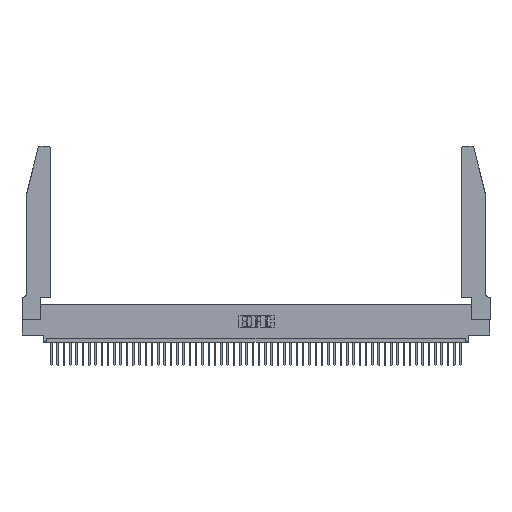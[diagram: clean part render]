
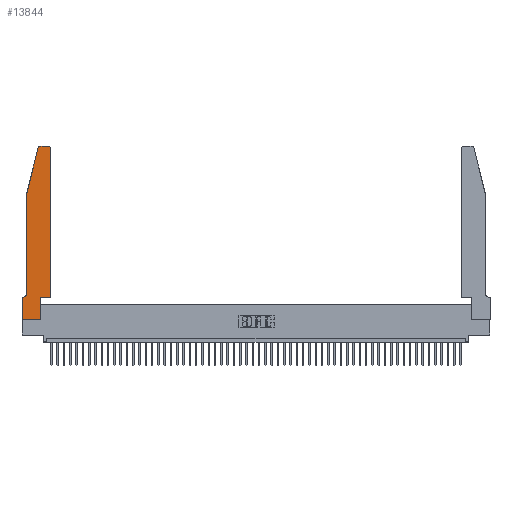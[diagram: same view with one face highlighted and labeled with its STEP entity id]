
A CAD part, top view. The second image highlights one B-rep face of the part: STEP entity #13844.
In plain terms, the highlighted planar face has unit normal (0, 0, 1).
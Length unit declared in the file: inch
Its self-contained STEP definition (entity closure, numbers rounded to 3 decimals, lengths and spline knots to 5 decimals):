
#1140 = VECTOR ( 'NONE', #16106, 39.37008 ) ;
#1264 = VERTEX_POINT ( 'NONE', #22103 ) ;
#1305 = DIRECTION ( 'NONE',  ( 0., 1., 0. ) ) ;
#1679 = CARTESIAN_POINT ( 'NONE',  ( 0.0755, 2., 0.37 ) ) ;
#2089 = DIRECTION ( 'NONE',  ( 0., 0., 1. ) ) ;
#2169 = DIRECTION ( 'NONE',  ( -1., 0., 0. ) ) ;
#2208 = DIRECTION ( 'NONE',  ( 0., 0., 1. ) ) ;
#2503 = VECTOR ( 'NONE', #2169, 39.37008 ) ;
#2646 = ORIENTED_EDGE ( 'NONE', *, *, #10434, .T. ) ;
#3497 = VERTEX_POINT ( 'NONE', #5968 ) ;
#3773 = DIRECTION ( 'NONE',  ( -1., 0., 0. ) ) ;
#3814 = ORIENTED_EDGE ( 'NONE', *, *, #42274, .T. ) ;
#4994 = VECTOR ( 'NONE', #3773, 39.37008 ) ;
#5667 = ORIENTED_EDGE ( 'NONE', *, *, #31963, .T. ) ;
#5926 = VERTEX_POINT ( 'NONE', #17185 ) ;
#5968 = CARTESIAN_POINT ( 'NONE',  ( 0., 0.35, 0.37 ) ) ;
#6052 = VERTEX_POINT ( 'NONE', #27589 ) ;
#6230 = VERTEX_POINT ( 'NONE', #17144 ) ;
#6250 = DIRECTION ( 'NONE',  ( 1., 0., 0. ) ) ;
#6266 = DIRECTION ( 'NONE',  ( 1., 0., 0. ) ) ;
#6328 = ORIENTED_EDGE ( 'NONE', *, *, #15241, .T. ) ;
#6505 = CARTESIAN_POINT ( 'NONE',  ( 0.2865, 0.35, 0.37 ) ) ;
#7185 = ORIENTED_EDGE ( 'NONE', *, *, #11481, .T. ) ;
#7549 = LINE ( 'NONE', #36276, #19295 ) ;
#8269 = ORIENTED_EDGE ( 'NONE', *, *, #35751, .T. ) ;
#8461 = EDGE_CURVE ( 'NONE', #5926, #13390, #28843, .T. ) ;
#9379 = CARTESIAN_POINT ( 'NONE',  ( 0.4505, 0.35, 0.37 ) ) ;
#10176 = VECTOR ( 'NONE', #50410, 39.37008 ) ;
#10383 = FACE_OUTER_BOUND ( 'NONE', #32331, .T. ) ;
#10434 = EDGE_CURVE ( 'NONE', #6052, #14651, #46537, .T. ) ;
#10548 = CARTESIAN_POINT ( 'NONE',  ( 0.4505, 0.35, 0.37 ) ) ;
#11481 = EDGE_CURVE ( 'NONE', #6230, #17994, #36032, .T. ) ;
#12273 = EDGE_CURVE ( 'NONE', #17994, #3497, #48941, .T. ) ;
#13036 = EDGE_CURVE ( 'NONE', #26309, #51332, #46368, .T. ) ;
#13390 = VERTEX_POINT ( 'NONE', #35674 ) ;
#13400 = VECTOR ( 'NONE', #46387, 39.37008 ) ;
#13844 = ADVANCED_FACE ( 'NONE', ( #10383 ), #34217, .T. ) ;
#13885 = ORIENTED_EDGE ( 'NONE', *, *, #8461, .T. ) ;
#14651 = VERTEX_POINT ( 'NONE', #30762 ) ;
#14690 = CARTESIAN_POINT ( 'NONE',  ( 0.0755, 2., 0.37 ) ) ;
#15241 = EDGE_CURVE ( 'NONE', #1264, #6230, #45476, .T. ) ;
#15530 = CARTESIAN_POINT ( 'NONE',  ( 0.2605, 2.75, 0.37 ) ) ;
#16106 = DIRECTION ( 'NONE',  ( 0., 1., 0. ) ) ;
#16199 = DIRECTION ( 'NONE',  ( 1., 0., 0. ) ) ;
#16653 = AXIS2_PLACEMENT_3D ( 'NONE', #29723, #2208, #18300 ) ;
#16791 = AXIS2_PLACEMENT_3D ( 'NONE', #39643, #2089, #6266 ) ;
#17144 = CARTESIAN_POINT ( 'NONE',  ( 0.0755, 0.42, 0.37 ) ) ;
#17185 = CARTESIAN_POINT ( 'NONE',  ( 0.4505, 2.72, 0.37 ) ) ;
#17994 = VERTEX_POINT ( 'NONE', #50939 ) ;
#18300 = DIRECTION ( 'NONE',  ( 1., 0., 0. ) ) ;
#19295 = VECTOR ( 'NONE', #16199, 39.37008 ) ;
#21128 = ORIENTED_EDGE ( 'NONE', *, *, #12273, .T. ) ;
#21629 = DIRECTION ( 'NONE',  ( -0.239, -0.971, 0. ) ) ;
#22103 = CARTESIAN_POINT ( 'NONE',  ( 0.0755, 2., 0.37 ) ) ;
#24107 = ORIENTED_EDGE ( 'NONE', *, *, #24255, .T. ) ;
#24255 = EDGE_CURVE ( 'NONE', #3497, #38694, #25208, .T. ) ;
#24711 = CARTESIAN_POINT ( 'NONE',  ( 0.2865, 0.35, 0.37 ) ) ;
#25208 = LINE ( 'NONE', #44828, #13400 ) ;
#25330 = VECTOR ( 'NONE', #6250, 39.37008 ) ;
#26196 = CARTESIAN_POINT ( 'NONE',  ( 0.284, 2.72, 0.37 ) ) ;
#26309 = VERTEX_POINT ( 'NONE', #6505 ) ;
#26932 = CARTESIAN_POINT ( 'NONE',  ( 0.2865, 0., 0.37 ) ) ;
#27589 = CARTESIAN_POINT ( 'NONE',  ( 0.284, 2.75, 0.37 ) ) ;
#28843 = CIRCLE ( 'NONE', #16791, 0.03 ) ;
#29723 = CARTESIAN_POINT ( 'NONE',  ( 0., 0.35, 0.37 ) ) ;
#30401 = LINE ( 'NONE', #15530, #4994 ) ;
#30762 = CARTESIAN_POINT ( 'NONE',  ( 0.25487, 2.72718, 0.37 ) ) ;
#31963 = EDGE_CURVE ( 'NONE', #14651, #1264, #38817, .T. ) ;
#32095 = LINE ( 'NONE', #24711, #34616 ) ;
#32331 = EDGE_LOOP ( 'NONE', ( #8269, #2646, #5667, #6328, #7185, #21128, #24107, #3814, #34316, #50699, #38748, #13885 ) ) ;
#32713 = CARTESIAN_POINT ( 'NONE',  ( 0.4505, 0.35, 0.37 ) ) ;
#34014 = LINE ( 'NONE', #32713, #1140 ) ;
#34217 = PLANE ( 'NONE',  #16653 ) ;
#34316 = ORIENTED_EDGE ( 'NONE', *, *, #48409, .T. ) ;
#34616 = VECTOR ( 'NONE', #1305, 39.37008 ) ;
#35076 = CARTESIAN_POINT ( 'NONE',  ( 0., 0., 0.37 ) ) ;
#35674 = CARTESIAN_POINT ( 'NONE',  ( 0.4205, 2.75, 0.37 ) ) ;
#35751 = EDGE_CURVE ( 'NONE', #13390, #6052, #30401, .T. ) ;
#36005 = DIRECTION ( 'NONE',  ( 0., 0., -1. ) ) ;
#36032 = CIRCLE ( 'NONE', #40713, 0.07 ) ;
#36276 = CARTESIAN_POINT ( 'NONE',  ( 0., 0., 0.37 ) ) ;
#36320 = VECTOR ( 'NONE', #21629, 39.37008 ) ;
#38347 = EDGE_CURVE ( 'NONE', #51332, #5926, #34014, .T. ) ;
#38694 = VERTEX_POINT ( 'NONE', #35076 ) ;
#38748 = ORIENTED_EDGE ( 'NONE', *, *, #38347, .T. ) ;
#38817 = LINE ( 'NONE', #1679, #36320 ) ;
#39643 = CARTESIAN_POINT ( 'NONE',  ( 0.4205, 2.72, 0.37 ) ) ;
#40713 = AXIS2_PLACEMENT_3D ( 'NONE', #44878, #36005, #46877 ) ;
#42274 = EDGE_CURVE ( 'NONE', #38694, #42616, #7549, .T. ) ;
#42616 = VERTEX_POINT ( 'NONE', #26932 ) ;
#44828 = CARTESIAN_POINT ( 'NONE',  ( 0., 0., 0.37 ) ) ;
#44878 = CARTESIAN_POINT ( 'NONE',  ( 0.0055, 0.42, 0.37 ) ) ;
#45476 = LINE ( 'NONE', #14690, #10176 ) ;
#46368 = LINE ( 'NONE', #10548, #25330 ) ;
#46387 = DIRECTION ( 'NONE',  ( 0., -1., 0. ) ) ;
#46537 = CIRCLE ( 'NONE', #48746, 0.03 ) ;
#46877 = DIRECTION ( 'NONE',  ( -1., 0., 0. ) ) ;
#48409 = EDGE_CURVE ( 'NONE', #42616, #26309, #32095, .T. ) ;
#48746 = AXIS2_PLACEMENT_3D ( 'NONE', #26196, #50092, #49564 ) ;
#48941 = LINE ( 'NONE', #49086, #2503 ) ;
#49086 = CARTESIAN_POINT ( 'NONE',  ( 0.0755, 0.35, 0.37 ) ) ;
#49564 = DIRECTION ( 'NONE',  ( 1., 0., 0. ) ) ;
#50092 = DIRECTION ( 'NONE',  ( 0., 0., 1. ) ) ;
#50410 = DIRECTION ( 'NONE',  ( 0., -1., 0. ) ) ;
#50699 = ORIENTED_EDGE ( 'NONE', *, *, #13036, .T. ) ;
#50939 = CARTESIAN_POINT ( 'NONE',  ( 0.0055, 0.35, 0.37 ) ) ;
#51332 = VERTEX_POINT ( 'NONE', #9379 ) ;
